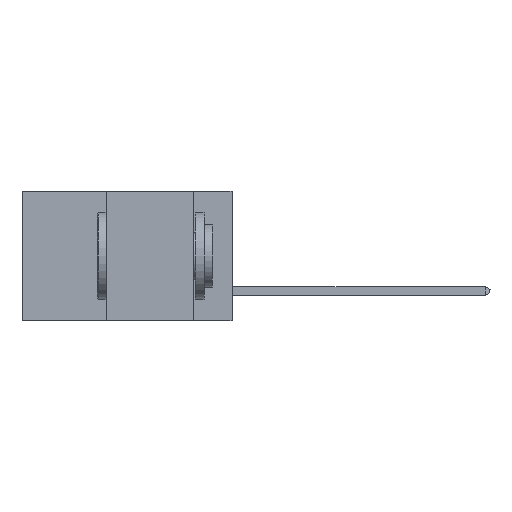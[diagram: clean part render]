
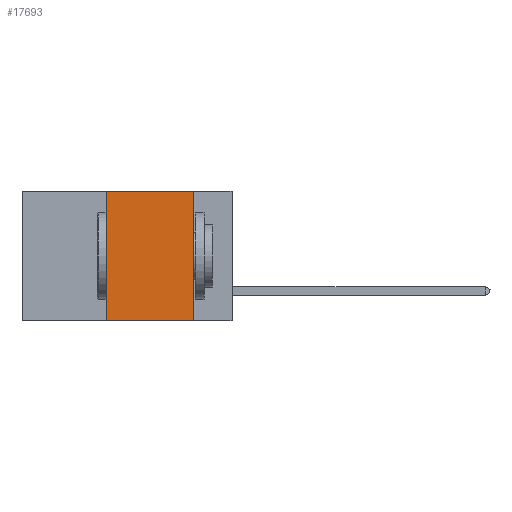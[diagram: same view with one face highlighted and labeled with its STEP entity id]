
A CAD part, left-side view. The second image highlights one B-rep face of the part: STEP entity #17693.
In plain terms, the highlighted planar face has unit normal (-1, 0, 0).
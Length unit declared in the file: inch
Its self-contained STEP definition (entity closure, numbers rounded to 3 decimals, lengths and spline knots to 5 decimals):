
#351 = VERTEX_POINT ( 'NONE', #14146 ) ;
#1418 = CARTESIAN_POINT ( 'NONE',  ( 0., 0.6, 0. ) ) ;
#3496 = LINE ( 'NONE', #20506, #23052 ) ;
#4951 = ORIENTED_EDGE ( 'NONE', *, *, #14132, .F. ) ;
#5499 = LINE ( 'NONE', #11666, #14859 ) ;
#7460 = VECTOR ( 'NONE', #8855, 39.37008 ) ;
#8561 = DIRECTION ( 'NONE',  ( 1., 0., 0. ) ) ;
#8855 = DIRECTION ( 'NONE',  ( 0., -1., 0. ) ) ;
#8917 = AXIS2_PLACEMENT_3D ( 'NONE', #1418, #8561, #21611 ) ;
#9472 = ORIENTED_EDGE ( 'NONE', *, *, #20673, .T. ) ;
#9698 = CARTESIAN_POINT ( 'NONE',  ( 0., 0.11, -0.37 ) ) ;
#9809 = FACE_OUTER_BOUND ( 'NONE', #13482, .T. ) ;
#10686 = LINE ( 'NONE', #20101, #7460 ) ;
#11666 = CARTESIAN_POINT ( 'NONE',  ( 0., 0.11, 0. ) ) ;
#11821 = CARTESIAN_POINT ( 'NONE',  ( 0., 0.6, -0.37 ) ) ;
#12758 = ORIENTED_EDGE ( 'NONE', *, *, #23270, .F. ) ;
#13482 = EDGE_LOOP ( 'NONE', ( #4951, #22010, #12758, #9472 ) ) ;
#14132 = EDGE_CURVE ( 'NONE', #20319, #23791, #5499, .T. ) ;
#14146 = CARTESIAN_POINT ( 'NONE',  ( 0., 0.36, -0.37 ) ) ;
#14859 = VECTOR ( 'NONE', #15739, 39.37008 ) ;
#15137 = LINE ( 'NONE', #11821, #15737 ) ;
#15737 = VECTOR ( 'NONE', #17543, 39.37008 ) ;
#15739 = DIRECTION ( 'NONE',  ( 0., 0., -1. ) ) ;
#16277 = PLANE ( 'NONE',  #8917 ) ;
#16704 = EDGE_CURVE ( 'NONE', #19230, #20319, #10686, .T. ) ;
#17261 = CARTESIAN_POINT ( 'NONE',  ( 0., 0.36, 0. ) ) ;
#17543 = DIRECTION ( 'NONE',  ( 0., -1., 0. ) ) ;
#17693 = ADVANCED_FACE ( 'NONE', ( #9809 ), #16277, .F. ) ;
#18662 = CARTESIAN_POINT ( 'NONE',  ( 0., 0.11, 0. ) ) ;
#19230 = VERTEX_POINT ( 'NONE', #17261 ) ;
#20101 = CARTESIAN_POINT ( 'NONE',  ( 0., 0.6, 0. ) ) ;
#20319 = VERTEX_POINT ( 'NONE', #18662 ) ;
#20506 = CARTESIAN_POINT ( 'NONE',  ( 0., 0.36, 0. ) ) ;
#20673 = EDGE_CURVE ( 'NONE', #351, #23791, #15137, .T. ) ;
#21611 = DIRECTION ( 'NONE',  ( 0., 0., -1. ) ) ;
#22010 = ORIENTED_EDGE ( 'NONE', *, *, #16704, .F. ) ;
#22375 = DIRECTION ( 'NONE',  ( 0., 0., 1. ) ) ;
#23052 = VECTOR ( 'NONE', #22375, 39.37008 ) ;
#23270 = EDGE_CURVE ( 'NONE', #351, #19230, #3496, .T. ) ;
#23791 = VERTEX_POINT ( 'NONE', #9698 ) ;
